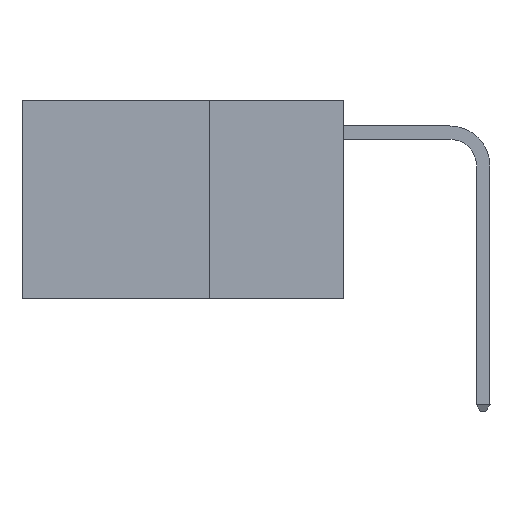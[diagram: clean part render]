
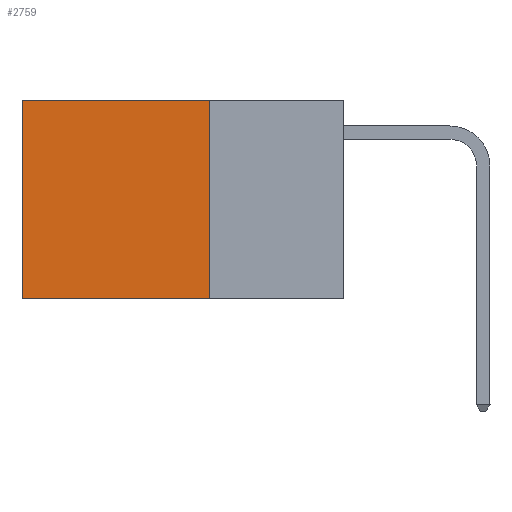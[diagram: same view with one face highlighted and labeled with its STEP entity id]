
A CAD part, left-side view. The second image highlights one B-rep face of the part: STEP entity #2759.
In plain terms, the highlighted planar face has unit normal (-1, 0, 0).
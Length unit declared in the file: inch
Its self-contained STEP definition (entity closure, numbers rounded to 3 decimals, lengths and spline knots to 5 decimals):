
#21 = LINE ( 'NONE', #13389, #5712 ) ;
#270 = EDGE_CURVE ( 'NONE', #22601, #14007, #1791, .T. ) ;
#286 = LINE ( 'NONE', #22540, #13237 ) ;
#610 = ORIENTED_EDGE ( 'NONE', *, *, #25154, .F. ) ;
#1117 = EDGE_LOOP ( 'NONE', ( #14822, #6498, #610, #27642 ) ) ;
#1363 = CARTESIAN_POINT ( 'NONE',  ( 0.2625, 0.25, 0. ) ) ;
#1791 = LINE ( 'NONE', #14341, #20349 ) ;
#1879 = LINE ( 'NONE', #25882, #21191 ) ;
#2759 = ADVANCED_FACE ( 'NONE', ( #24655 ), #11109, .F. ) ;
#3806 = DIRECTION ( 'NONE',  ( 1., 0., 0. ) ) ;
#5712 = VECTOR ( 'NONE', #27709, 39.37008 ) ;
#6498 = ORIENTED_EDGE ( 'NONE', *, *, #19303, .F. ) ;
#8518 = VERTEX_POINT ( 'NONE', #12913 ) ;
#9367 = AXIS2_PLACEMENT_3D ( 'NONE', #1363, #3806, #20735 ) ;
#11109 = PLANE ( 'NONE',  #9367 ) ;
#11545 = DIRECTION ( 'NONE',  ( 0., 1., 0. ) ) ;
#12913 = CARTESIAN_POINT ( 'NONE',  ( 0.2625, 0.25, -0.37 ) ) ;
#13007 = CARTESIAN_POINT ( 'NONE',  ( 0.2625, 0.6, 0. ) ) ;
#13237 = VECTOR ( 'NONE', #27230, 39.37008 ) ;
#13389 = CARTESIAN_POINT ( 'NONE',  ( 0.2625, 0.25, 0. ) ) ;
#14007 = VERTEX_POINT ( 'NONE', #18147 ) ;
#14341 = CARTESIAN_POINT ( 'NONE',  ( 0.2625, 0.6, 0. ) ) ;
#14822 = ORIENTED_EDGE ( 'NONE', *, *, #270, .T. ) ;
#16783 = DIRECTION ( 'NONE',  ( 0., 0., -1. ) ) ;
#17362 = EDGE_CURVE ( 'NONE', #21686, #22601, #286, .T. ) ;
#18147 = CARTESIAN_POINT ( 'NONE',  ( 0.2625, 0.6, -0.37 ) ) ;
#19303 = EDGE_CURVE ( 'NONE', #8518, #14007, #1879, .T. ) ;
#20349 = VECTOR ( 'NONE', #16783, 39.37008 ) ;
#20735 = DIRECTION ( 'NONE',  ( 0., 0., -1. ) ) ;
#21191 = VECTOR ( 'NONE', #11545, 39.37008 ) ;
#21686 = VERTEX_POINT ( 'NONE', #23944 ) ;
#22540 = CARTESIAN_POINT ( 'NONE',  ( 0.2625, 0.25, 0. ) ) ;
#22601 = VERTEX_POINT ( 'NONE', #13007 ) ;
#23944 = CARTESIAN_POINT ( 'NONE',  ( 0.2625, 0.25, 0. ) ) ;
#24655 = FACE_OUTER_BOUND ( 'NONE', #1117, .T. ) ;
#25154 = EDGE_CURVE ( 'NONE', #21686, #8518, #21, .T. ) ;
#25882 = CARTESIAN_POINT ( 'NONE',  ( 0.2625, 0.25, -0.37 ) ) ;
#27230 = DIRECTION ( 'NONE',  ( 0., 1., 0. ) ) ;
#27642 = ORIENTED_EDGE ( 'NONE', *, *, #17362, .T. ) ;
#27709 = DIRECTION ( 'NONE',  ( 0., 0., -1. ) ) ;
